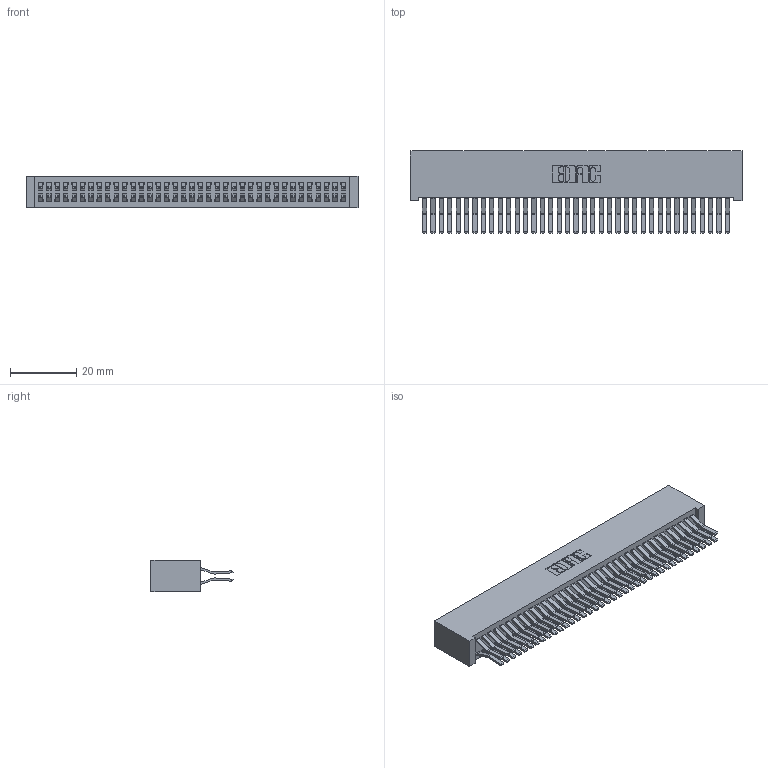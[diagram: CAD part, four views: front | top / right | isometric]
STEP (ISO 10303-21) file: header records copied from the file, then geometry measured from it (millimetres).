
FILE_DESCRIPTION (( 'STEP AP203' ), '1' );
FILE_NAME ('342-074-560-201.STEP', '2018-08-13T11:56:06', ( '' ), ( '' ), 'SwSTEP 2.0', 'SolidWorks 2016', '' );
FILE_SCHEMA (( 'CONFIG_CONTROL_DESIGN' ));
Length unit declared in the file: inch
Products named in the file (3): 342 Part_Lugless; 345-292-001_560 Tail; 342-074-560-201
Assembly tree (75 placements, depth 2):
  342-074-560-201
    342 Part_Lugless
    345-292-001_560 Tail  x74
Bounding box: 100.23 x 24.78 x 9.4 mm (x, y, z)
Volume: 9907.2 mm3; surface area: 17614.4 mm2
Topology: 75 solids, 75 shells, 4098 faces, 12189 edges, 8026 vertices
Faces by surface type: plane 2726, cylinder 1372
Entity records: 24129 total; most frequent: CARTESIAN_POINT 4002, ORIENTED_EDGE 3938, DIRECTION 3425, EDGE_CURVE 1969, LINE 1845, VECTOR 1845, VERTEX_POINT 1310, AXIS2_PLACEMENT_3D 790
